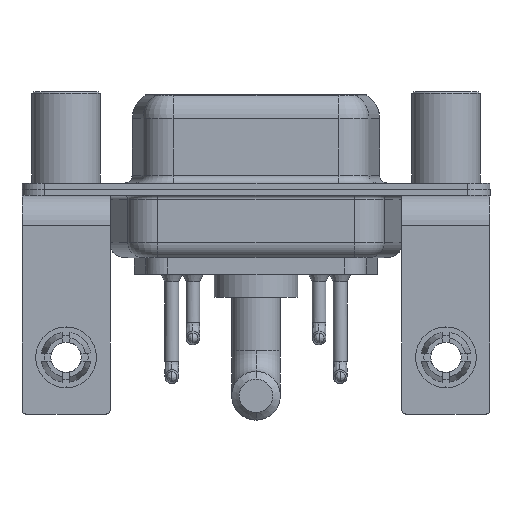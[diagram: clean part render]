
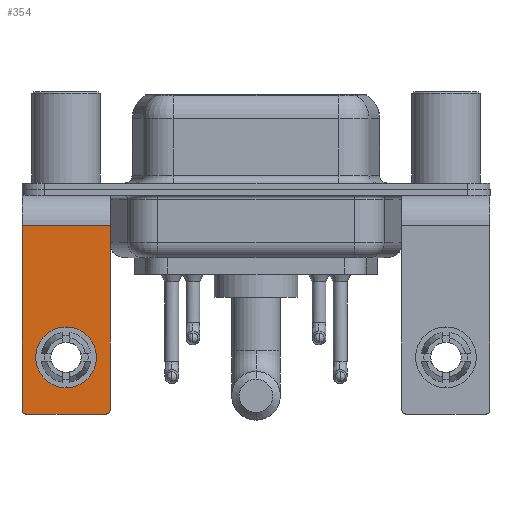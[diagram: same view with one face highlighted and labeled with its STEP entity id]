
A CAD part, front view. The second image highlights one B-rep face of the part: STEP entity #354.
In plain terms, the highlighted planar face has unit normal (0, -1, 0).
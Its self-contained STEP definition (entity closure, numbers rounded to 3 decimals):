
#328 = CARTESIAN_POINT ( 'NONE',  ( -2.65, -6.25, -14.8 ) ) ;
#354 = ADVANCED_FACE ( 'NONE', ( #4315, #9403 ), #17243, .F. ) ;
#371 = DIRECTION ( 'NONE',  ( 0., 1., 0. ) ) ;
#379 = VERTEX_POINT ( 'NONE', #7793 ) ;
#390 = CARTESIAN_POINT ( 'NONE',  ( 2.9, -6.25, -2.4 ) ) ;
#989 = VECTOR ( 'NONE', #17614, 1000. ) ;
#1055 = ORIENTED_EDGE ( 'NONE', *, *, #1884, .T. ) ;
#1162 = CARTESIAN_POINT ( 'NONE',  ( -2.9, -6.25, -2.4 ) ) ;
#1224 = CARTESIAN_POINT ( 'NONE',  ( -2.65, -6.25, -14.55 ) ) ;
#1884 = EDGE_CURVE ( 'NONE', #3670, #18450, #12290, .T. ) ;
#2044 = VERTEX_POINT ( 'NONE', #328 ) ;
#2365 = EDGE_LOOP ( 'NONE', ( #13399, #9580, #16732, #8570, #10451, #13692 ) ) ;
#2543 = AXIS2_PLACEMENT_3D ( 'NONE', #6036, #12239, #5740 ) ;
#2761 = CARTESIAN_POINT ( 'NONE',  ( -2.9, -6.25, -14.55 ) ) ;
#3273 = DIRECTION ( 'NONE',  ( 0., 0., 1. ) ) ;
#3641 = AXIS2_PLACEMENT_3D ( 'NONE', #4741, #16602, #10672 ) ;
#3670 = VERTEX_POINT ( 'NONE', #16687 ) ;
#4315 = FACE_BOUND ( 'NONE', #7266, .T. ) ;
#4640 = DIRECTION ( 'NONE',  ( -1., 0., 0. ) ) ;
#4741 = CARTESIAN_POINT ( 'NONE',  ( 0., -6.25, -11.07 ) ) ;
#4923 = AXIS2_PLACEMENT_3D ( 'NONE', #1224, #10453, #16583 ) ;
#4944 = LINE ( 'NONE', #12263, #12410 ) ;
#5484 = AXIS2_PLACEMENT_3D ( 'NONE', #6401, #371, #3273 ) ;
#5740 = DIRECTION ( 'NONE',  ( 0., 0., 1. ) ) ;
#5949 = VERTEX_POINT ( 'NONE', #2761 ) ;
#5954 = CARTESIAN_POINT ( 'NONE',  ( 0., -6.25, -9.07 ) ) ;
#5957 = EDGE_CURVE ( 'NONE', #16758, #5949, #8800, .T. ) ;
#6036 = CARTESIAN_POINT ( 'NONE',  ( 2.65, -6.25, -14.55 ) ) ;
#6401 = CARTESIAN_POINT ( 'NONE',  ( 2.9, -6.25, -2.4 ) ) ;
#6753 = CIRCLE ( 'NONE', #11564, 2. ) ;
#6782 = CARTESIAN_POINT ( 'NONE',  ( 2.9, -6.25, -2.4 ) ) ;
#7209 = EDGE_CURVE ( 'NONE', #18450, #3670, #6753, .T. ) ;
#7266 = EDGE_LOOP ( 'NONE', ( #1055, #9455 ) ) ;
#7718 = LINE ( 'NONE', #390, #17450 ) ;
#7793 = CARTESIAN_POINT ( 'NONE',  ( 2.65, -6.25, -14.8 ) ) ;
#8570 = ORIENTED_EDGE ( 'NONE', *, *, #13160, .T. ) ;
#8774 = CIRCLE ( 'NONE', #4923, 0.25 ) ;
#8800 = LINE ( 'NONE', #1162, #13067 ) ;
#9356 = EDGE_CURVE ( 'NONE', #379, #2044, #4944, .T. ) ;
#9403 = FACE_OUTER_BOUND ( 'NONE', #2365, .T. ) ;
#9455 = ORIENTED_EDGE ( 'NONE', *, *, #7209, .T. ) ;
#9580 = ORIENTED_EDGE ( 'NONE', *, *, #17242, .T. ) ;
#9984 = LINE ( 'NONE', #6782, #989 ) ;
#10191 = DIRECTION ( 'NONE',  ( 0., 0., -1. ) ) ;
#10451 = ORIENTED_EDGE ( 'NONE', *, *, #18985, .F. ) ;
#10453 = DIRECTION ( 'NONE',  ( 0., -1., 0. ) ) ;
#10672 = DIRECTION ( 'NONE',  ( 0., 0., 1. ) ) ;
#11564 = AXIS2_PLACEMENT_3D ( 'NONE', #17452, #17737, #18960 ) ;
#12239 = DIRECTION ( 'NONE',  ( 0., -1., 0. ) ) ;
#12263 = CARTESIAN_POINT ( 'NONE',  ( 2.9, -6.25, -14.8 ) ) ;
#12290 = CIRCLE ( 'NONE', #3641, 2. ) ;
#12410 = VECTOR ( 'NONE', #4640, 1000. ) ;
#13067 = VECTOR ( 'NONE', #10191, 1000. ) ;
#13160 = EDGE_CURVE ( 'NONE', #379, #17586, #17585, .T. ) ;
#13350 = CARTESIAN_POINT ( 'NONE',  ( 2.9, -6.25, -2.4 ) ) ;
#13399 = ORIENTED_EDGE ( 'NONE', *, *, #5957, .T. ) ;
#13692 = ORIENTED_EDGE ( 'NONE', *, *, #14108, .T. ) ;
#13837 = DIRECTION ( 'NONE',  ( 0., 0., -1. ) ) ;
#14108 = EDGE_CURVE ( 'NONE', #18893, #16758, #9984, .T. ) ;
#15288 = CARTESIAN_POINT ( 'NONE',  ( -2.9, -6.25, -2.4 ) ) ;
#16583 = DIRECTION ( 'NONE',  ( 0., 0., 1. ) ) ;
#16602 = DIRECTION ( 'NONE',  ( 0., 1., 0. ) ) ;
#16687 = CARTESIAN_POINT ( 'NONE',  ( 0., -6.25, -13.07 ) ) ;
#16732 = ORIENTED_EDGE ( 'NONE', *, *, #9356, .F. ) ;
#16758 = VERTEX_POINT ( 'NONE', #15288 ) ;
#17242 = EDGE_CURVE ( 'NONE', #5949, #2044, #8774, .T. ) ;
#17243 = PLANE ( 'NONE',  #5484 ) ;
#17450 = VECTOR ( 'NONE', #13837, 1000. ) ;
#17452 = CARTESIAN_POINT ( 'NONE',  ( 0., -6.25, -11.07 ) ) ;
#17585 = CIRCLE ( 'NONE', #2543, 0.25 ) ;
#17586 = VERTEX_POINT ( 'NONE', #19366 ) ;
#17614 = DIRECTION ( 'NONE',  ( -1., 0., 0. ) ) ;
#17737 = DIRECTION ( 'NONE',  ( 0., 1., 0. ) ) ;
#18450 = VERTEX_POINT ( 'NONE', #5954 ) ;
#18893 = VERTEX_POINT ( 'NONE', #13350 ) ;
#18960 = DIRECTION ( 'NONE',  ( 0., 0., 1. ) ) ;
#18985 = EDGE_CURVE ( 'NONE', #18893, #17586, #7718, .T. ) ;
#19366 = CARTESIAN_POINT ( 'NONE',  ( 2.9, -6.25, -14.55 ) ) ;
